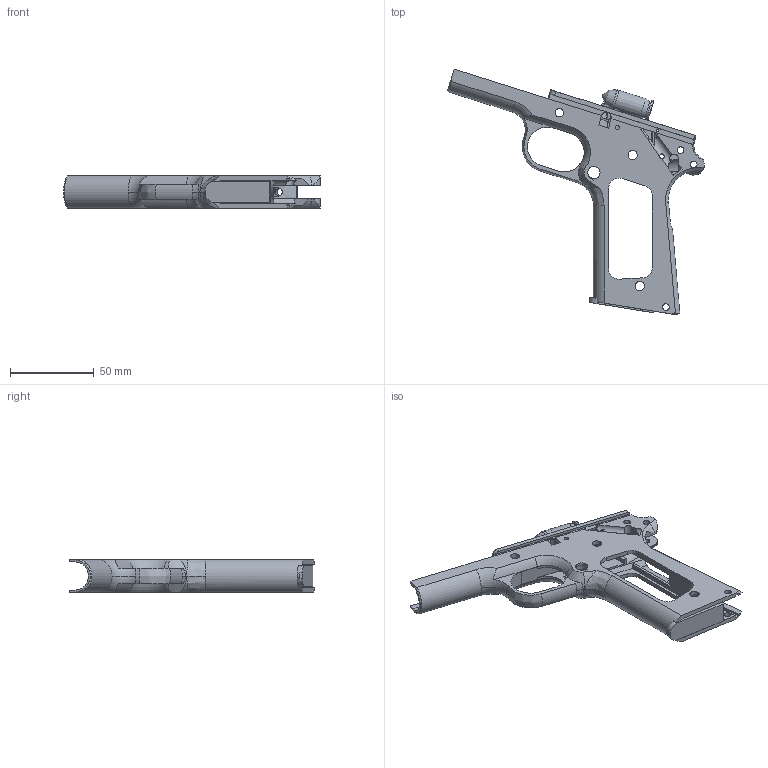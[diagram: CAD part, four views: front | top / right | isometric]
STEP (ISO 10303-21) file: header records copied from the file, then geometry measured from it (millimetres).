
FILE_DESCRIPTION((''),'2;1');
FILE_NAME('1911 GM Magazine Assy.stp','2011-11-23T20:47:36',('Bob'),(''),'Autodesk Inventor 2011','Autodesk Inventor 2011','');
FILE_SCHEMA(('AUTOMOTIVE_DESIGN { 1 0 10303 214 1 1 1 1 }'));
Length unit declared in the file: inch
Products named in the file (6): 1911 GM Magazine Assy; Magazine Body; Magazine Follower; Magazine Base Plate; 1911 Receiver; 45 ACP Cartridge
Assembly tree (5 placements, depth 2):
  1911 GM Magazine Assy
    Magazine Body
    Magazine Follower
    Magazine Base Plate
    1911 Receiver
    45 ACP Cartridge
Bounding box: 152.85 x 146.2 x 19.1 mm (x, y, z)
Volume: 45469.1 mm3; surface area: 39444.5 mm2
Topology: 5 solids, 5 shells, 305 faces, 925 edges, 614 vertices
Faces by surface type: plane 141, cylinder 113, cone 22, torus 16, bspline 13
Full cylindrical faces by diameter (mm): 1.575 x1, 1.588 x4, 2.451 x1, 2.51 x1, 2.794 x2, 3.175 x1, 3.957 x2, 3.988 x2, 4.001 x2, 4.166 x1, 4.724 x1, 4.775 x2, 5.105 x2, 5.537 x4, 5.556 x1, 7.315 x1, 7.938 x1, 10.16 x1, 12.019 x1, 12.726 x1
Entity records: 11265 total; most frequent: CARTESIAN_POINT 2793, DIRECTION 1723, ORIENTED_EDGE 1714, EDGE_CURVE 857, AXIS2_PLACEMENT_3D 648, VERTEX_POINT 604, VECTOR 427, LINE 427
